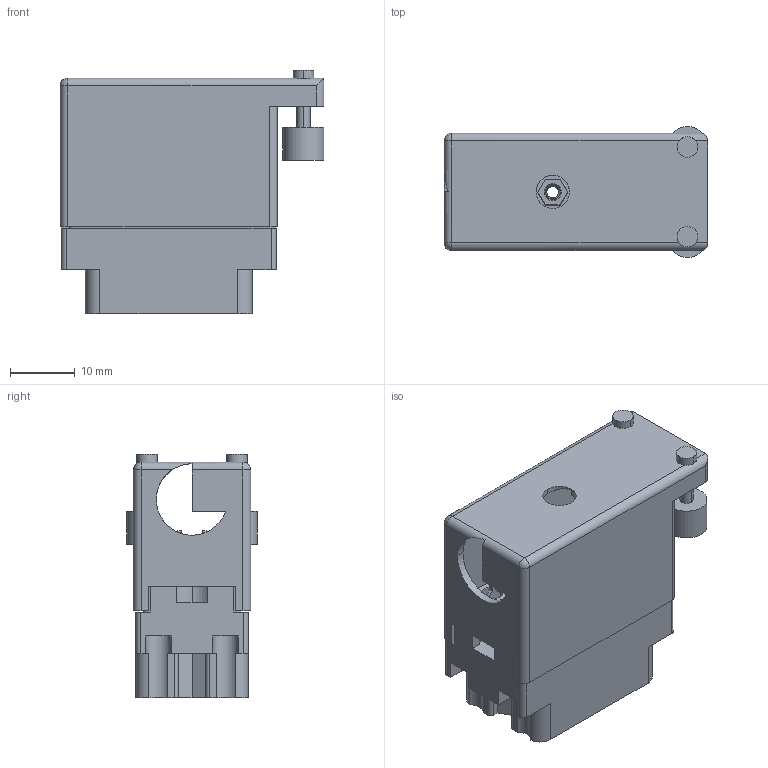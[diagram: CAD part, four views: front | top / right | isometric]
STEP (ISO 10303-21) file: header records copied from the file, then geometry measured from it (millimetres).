
FILE_DESCRIPTION (( 'STEP AP203' ), '1' );
FILE_NAME ('516-020-520-526.STEP', '2020-03-09T16:26:03', ( '' ), ( '' ), 'SwSTEP 2.0', 'SolidWorks 2016', '' );
FILE_SCHEMA (( 'CONFIG_CONTROL_DESIGN' ));
Length unit declared in the file: inch
Products named in the file (5): 516-292-001_520 Contact; 516 Plug Insulator_020; 516-252-025-100_516-252-025-100; 516-230-001_Plastic - 020 Side Entry; 516-020-520-526
Assembly tree (23 placements, depth 2):
  516-020-520-526
    516 Plug Insulator_020
    516-292-001_520 Contact  x20
    516-230-001_Plastic - 020 Side Entry
    516-252-025-100_516-252-025-100
Bounding box: 40.87 x 20.24 x 37.77 mm (x, y, z)
Volume: 8862.3 mm3; surface area: 16631.7 mm2
Topology: 23 solids, 23 shells, 2175 faces, 6305 edges, 4180 vertices
Faces by surface type: plane 1317, cylinder 722, bspline 123, cone 11, sphere 2
Entity records: 30710 total; most frequent: CARTESIAN_POINT 7808, ORIENTED_EDGE 4702, DIRECTION 4485, EDGE_CURVE 2351, LINE 1667, VECTOR 1667, VERTEX_POINT 1558, AXIS2_PLACEMENT_3D 1409
